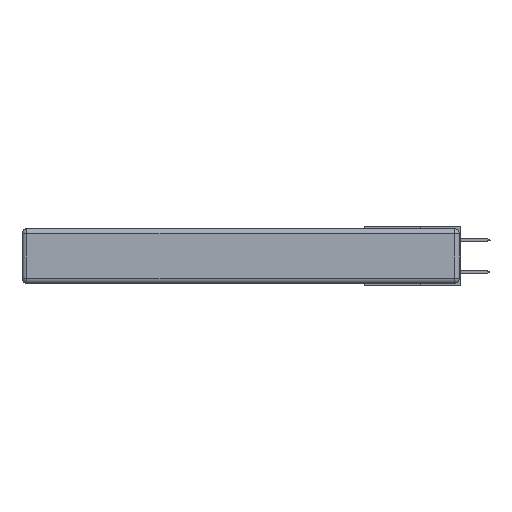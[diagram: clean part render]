
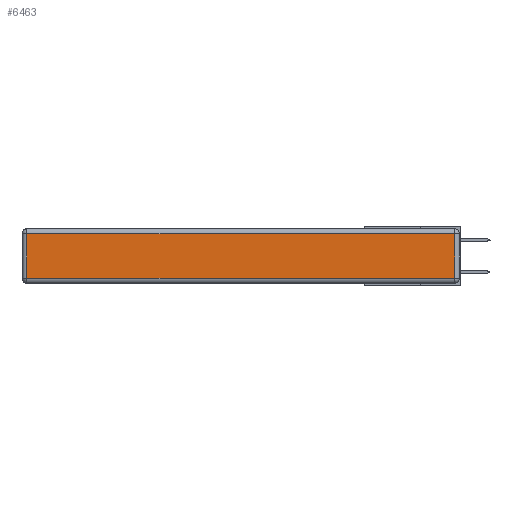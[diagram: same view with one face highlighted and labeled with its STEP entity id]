
A CAD part, left-side view. The second image highlights one B-rep face of the part: STEP entity #6463.
In plain terms, the highlighted planar face has unit normal (-1, 0, 0).
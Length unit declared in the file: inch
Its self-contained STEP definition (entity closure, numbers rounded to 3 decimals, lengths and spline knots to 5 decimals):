
#930 = ORIENTED_EDGE ( 'NONE', *, *, #5437, .T. ) ;
#2386 = VERTEX_POINT ( 'NONE', #28095 ) ;
#3059 = CARTESIAN_POINT ( 'NONE',  ( 0., 2.75, -0.03 ) ) ;
#3884 = VERTEX_POINT ( 'NONE', #30053 ) ;
#4301 = LINE ( 'NONE', #3059, #25641 ) ;
#5182 = ORIENTED_EDGE ( 'NONE', *, *, #27707, .T. ) ;
#5364 = ORIENTED_EDGE ( 'NONE', *, *, #9900, .T. ) ;
#5437 = EDGE_CURVE ( 'NONE', #2386, #14385, #7362, .T. ) ;
#5680 = DIRECTION ( 'NONE',  ( -1., 0., 0. ) ) ;
#6116 = DIRECTION ( 'NONE',  ( 0., -1., 0. ) ) ;
#6463 = ADVANCED_FACE ( 'NONE', ( #12087 ), #25274, .T. ) ;
#6688 = CARTESIAN_POINT ( 'NONE',  ( 0., 0.03, -0.343 ) ) ;
#7137 = VECTOR ( 'NONE', #6116, 39.37008 ) ;
#7362 = LINE ( 'NONE', #6688, #13016 ) ;
#7542 = VECTOR ( 'NONE', #33246, 39.37008 ) ;
#8410 = LINE ( 'NONE', #13768, #7542 ) ;
#9900 = EDGE_CURVE ( 'NONE', #14385, #3884, #4301, .T. ) ;
#11903 = ORIENTED_EDGE ( 'NONE', *, *, #12754, .T. ) ;
#12087 = FACE_OUTER_BOUND ( 'NONE', #32068, .T. ) ;
#12754 = EDGE_CURVE ( 'NONE', #32924, #2386, #25858, .T. ) ;
#13016 = VECTOR ( 'NONE', #13118, 39.37008 ) ;
#13118 = DIRECTION ( 'NONE',  ( 0., 0., 1. ) ) ;
#13768 = CARTESIAN_POINT ( 'NONE',  ( 0., 2.72, -0.343 ) ) ;
#14385 = VERTEX_POINT ( 'NONE', #14636 ) ;
#14636 = CARTESIAN_POINT ( 'NONE',  ( 0., 0.03, -0.03 ) ) ;
#16709 = AXIS2_PLACEMENT_3D ( 'NONE', #16992, #5680, #27951 ) ;
#16992 = CARTESIAN_POINT ( 'NONE',  ( 0., 0., -0.343 ) ) ;
#22528 = DIRECTION ( 'NONE',  ( 0., 1., 0. ) ) ;
#22802 = CARTESIAN_POINT ( 'NONE',  ( 0., 0., -0.313 ) ) ;
#25274 = PLANE ( 'NONE',  #16709 ) ;
#25641 = VECTOR ( 'NONE', #22528, 39.37008 ) ;
#25858 = LINE ( 'NONE', #22802, #7137 ) ;
#27707 = EDGE_CURVE ( 'NONE', #3884, #32924, #8410, .T. ) ;
#27951 = DIRECTION ( 'NONE',  ( 0., 0., 1. ) ) ;
#28095 = CARTESIAN_POINT ( 'NONE',  ( 0., 0.03, -0.313 ) ) ;
#28435 = CARTESIAN_POINT ( 'NONE',  ( 0., 2.72, -0.313 ) ) ;
#30053 = CARTESIAN_POINT ( 'NONE',  ( 0., 2.72, -0.03 ) ) ;
#32068 = EDGE_LOOP ( 'NONE', ( #11903, #930, #5364, #5182 ) ) ;
#32924 = VERTEX_POINT ( 'NONE', #28435 ) ;
#33246 = DIRECTION ( 'NONE',  ( 0., 0., -1. ) ) ;
